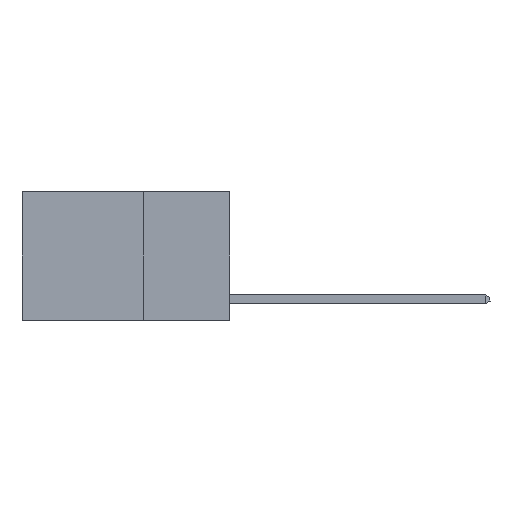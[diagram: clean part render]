
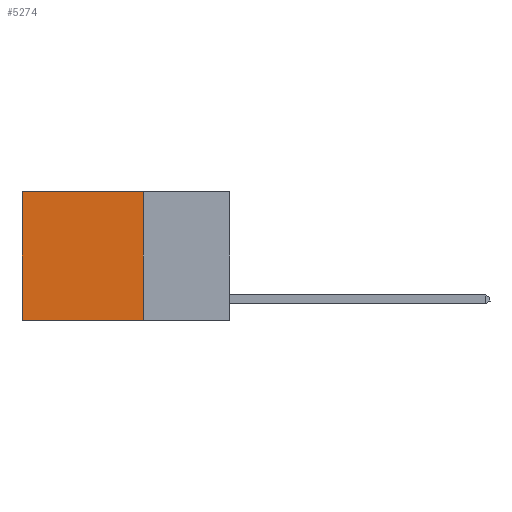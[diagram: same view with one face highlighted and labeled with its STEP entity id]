
A CAD part, left-side view. The second image highlights one B-rep face of the part: STEP entity #5274.
In plain terms, the highlighted planar face has unit normal (-1, 0, 0).
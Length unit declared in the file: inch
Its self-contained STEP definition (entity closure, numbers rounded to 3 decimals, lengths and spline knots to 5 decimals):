
#82 = EDGE_CURVE ( 'NONE', #10730, #11441, #11068, .T. ) ;
#192 = PLANE ( 'NONE',  #1145 ) ;
#491 = VECTOR ( 'NONE', #2992, 39.37008 ) ;
#782 = VECTOR ( 'NONE', #9209, 39.37008 ) ;
#1145 = AXIS2_PLACEMENT_3D ( 'NONE', #11679, #3454, #8576 ) ;
#1410 = CARTESIAN_POINT ( 'NONE',  ( 0.2625, 0.6, 0. ) ) ;
#2992 = DIRECTION ( 'NONE',  ( 0., 1., 0. ) ) ;
#3056 = CARTESIAN_POINT ( 'NONE',  ( 0.2625, 0.25, 0. ) ) ;
#3069 = CARTESIAN_POINT ( 'NONE',  ( 0.2625, 0.6, 0. ) ) ;
#3454 = DIRECTION ( 'NONE',  ( 1., 0., 0. ) ) ;
#3463 = DIRECTION ( 'NONE',  ( 0., 1., 0. ) ) ;
#3722 = LINE ( 'NONE', #3056, #782 ) ;
#3877 = EDGE_CURVE ( 'NONE', #10502, #6015, #4478, .T. ) ;
#4129 = ORIENTED_EDGE ( 'NONE', *, *, #10437, .T. ) ;
#4478 = LINE ( 'NONE', #10794, #12096 ) ;
#5274 = ADVANCED_FACE ( 'NONE', ( #10405 ), #192, .F. ) ;
#5995 = CARTESIAN_POINT ( 'NONE',  ( 0.2625, 0.25, 0. ) ) ;
#6015 = VERTEX_POINT ( 'NONE', #9239 ) ;
#6081 = CARTESIAN_POINT ( 'NONE',  ( 0.2625, 0.25, -0.37 ) ) ;
#6209 = VECTOR ( 'NONE', #12507, 39.37008 ) ;
#6790 = ORIENTED_EDGE ( 'NONE', *, *, #82, .T. ) ;
#8150 = EDGE_CURVE ( 'NONE', #10730, #10502, #3722, .T. ) ;
#8576 = DIRECTION ( 'NONE',  ( 0., 0., -1. ) ) ;
#9209 = DIRECTION ( 'NONE',  ( 0., 0., -1. ) ) ;
#9239 = CARTESIAN_POINT ( 'NONE',  ( 0.2625, 0.6, -0.37 ) ) ;
#10068 = ORIENTED_EDGE ( 'NONE', *, *, #8150, .F. ) ;
#10405 = FACE_OUTER_BOUND ( 'NONE', #12312, .T. ) ;
#10437 = EDGE_CURVE ( 'NONE', #11441, #6015, #13343, .T. ) ;
#10502 = VERTEX_POINT ( 'NONE', #6081 ) ;
#10730 = VERTEX_POINT ( 'NONE', #5995 ) ;
#10794 = CARTESIAN_POINT ( 'NONE',  ( 0.2625, 0.25, -0.37 ) ) ;
#11068 = LINE ( 'NONE', #12244, #491 ) ;
#11387 = ORIENTED_EDGE ( 'NONE', *, *, #3877, .F. ) ;
#11441 = VERTEX_POINT ( 'NONE', #1410 ) ;
#11679 = CARTESIAN_POINT ( 'NONE',  ( 0.2625, 0.25, 0. ) ) ;
#12096 = VECTOR ( 'NONE', #3463, 39.37008 ) ;
#12244 = CARTESIAN_POINT ( 'NONE',  ( 0.2625, 0.25, 0. ) ) ;
#12312 = EDGE_LOOP ( 'NONE', ( #4129, #11387, #10068, #6790 ) ) ;
#12507 = DIRECTION ( 'NONE',  ( 0., 0., -1. ) ) ;
#13343 = LINE ( 'NONE', #3069, #6209 ) ;
